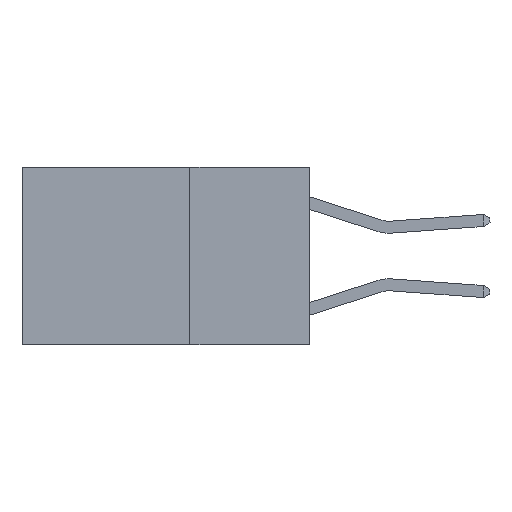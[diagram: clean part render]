
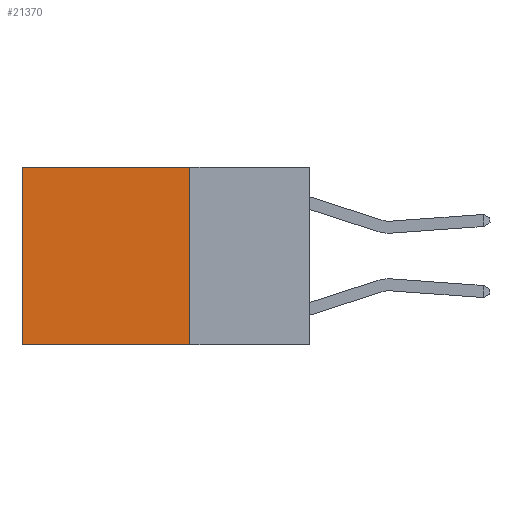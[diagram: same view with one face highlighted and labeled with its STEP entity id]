
A CAD part, left-side view. The second image highlights one B-rep face of the part: STEP entity #21370.
In plain terms, the highlighted planar face has unit normal (-1, 0, 0).
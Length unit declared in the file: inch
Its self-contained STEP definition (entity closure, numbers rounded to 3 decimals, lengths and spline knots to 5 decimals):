
#194 = DIRECTION ( 'NONE',  ( 0., 1., 0. ) ) ;
#407 = LINE ( 'NONE', #4720, #4729 ) ;
#1599 = DIRECTION ( 'NONE',  ( 1., 0., 0. ) ) ;
#1604 = EDGE_CURVE ( 'NONE', #9232, #16816, #22306, .T. ) ;
#1682 = DIRECTION ( 'NONE',  ( 0., 0., -1. ) ) ;
#2153 = LINE ( 'NONE', #20014, #10791 ) ;
#2515 = DIRECTION ( 'NONE',  ( 0., 0., -1. ) ) ;
#4720 = CARTESIAN_POINT ( 'NONE',  ( 0.2625, 0.25, 0. ) ) ;
#4729 = VECTOR ( 'NONE', #19392, 39.37008 ) ;
#4908 = CARTESIAN_POINT ( 'NONE',  ( 0.2625, 0.25, -0.37 ) ) ;
#5401 = ORIENTED_EDGE ( 'NONE', *, *, #6130, .T. ) ;
#5518 = FACE_OUTER_BOUND ( 'NONE', #17017, .T. ) ;
#6130 = EDGE_CURVE ( 'NONE', #22151, #19457, #407, .T. ) ;
#6843 = DIRECTION ( 'NONE',  ( 0., 0., -1. ) ) ;
#8003 = EDGE_CURVE ( 'NONE', #22151, #9232, #21774, .T. ) ;
#8779 = CARTESIAN_POINT ( 'NONE',  ( 0.2625, 0.6, 0. ) ) ;
#9232 = VERTEX_POINT ( 'NONE', #4908 ) ;
#9682 = CARTESIAN_POINT ( 'NONE',  ( 0.2625, 0.25, 0. ) ) ;
#9776 = AXIS2_PLACEMENT_3D ( 'NONE', #23590, #1599, #1682 ) ;
#10791 = VECTOR ( 'NONE', #6843, 39.37008 ) ;
#11284 = CARTESIAN_POINT ( 'NONE',  ( 0.2625, 0.25, -0.37 ) ) ;
#12503 = VECTOR ( 'NONE', #194, 39.37008 ) ;
#13390 = CARTESIAN_POINT ( 'NONE',  ( 0.2625, 0.25, 0. ) ) ;
#16554 = EDGE_CURVE ( 'NONE', #19457, #16816, #2153, .T. ) ;
#16816 = VERTEX_POINT ( 'NONE', #18927 ) ;
#17017 = EDGE_LOOP ( 'NONE', ( #17861, #20873, #17089, #5401 ) ) ;
#17089 = ORIENTED_EDGE ( 'NONE', *, *, #8003, .F. ) ;
#17861 = ORIENTED_EDGE ( 'NONE', *, *, #16554, .T. ) ;
#18927 = CARTESIAN_POINT ( 'NONE',  ( 0.2625, 0.6, -0.37 ) ) ;
#19392 = DIRECTION ( 'NONE',  ( 0., 1., 0. ) ) ;
#19457 = VERTEX_POINT ( 'NONE', #8779 ) ;
#20014 = CARTESIAN_POINT ( 'NONE',  ( 0.2625, 0.6, 0. ) ) ;
#20873 = ORIENTED_EDGE ( 'NONE', *, *, #1604, .F. ) ;
#21370 = ADVANCED_FACE ( 'NONE', ( #5518 ), #23444, .F. ) ;
#21774 = LINE ( 'NONE', #9682, #23242 ) ;
#22151 = VERTEX_POINT ( 'NONE', #13390 ) ;
#22306 = LINE ( 'NONE', #11284, #12503 ) ;
#23242 = VECTOR ( 'NONE', #2515, 39.37008 ) ;
#23444 = PLANE ( 'NONE',  #9776 ) ;
#23590 = CARTESIAN_POINT ( 'NONE',  ( 0.2625, 0.25, 0. ) ) ;
